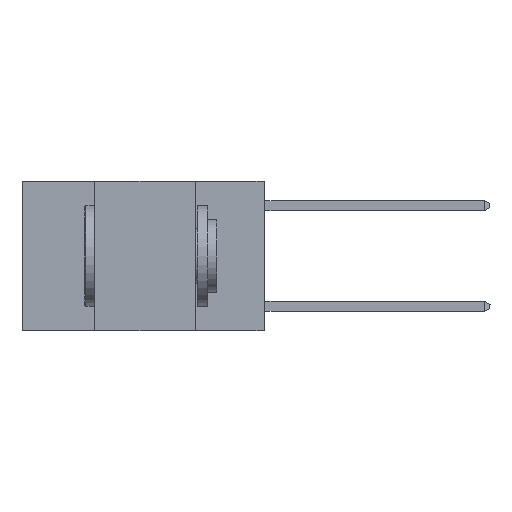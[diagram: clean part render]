
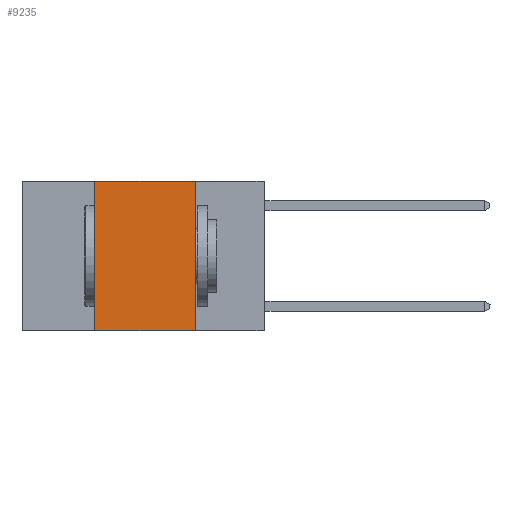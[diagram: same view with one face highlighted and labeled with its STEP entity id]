
A CAD part, left-side view. The second image highlights one B-rep face of the part: STEP entity #9235.
In plain terms, the highlighted planar face has unit normal (-1, 0, 0).
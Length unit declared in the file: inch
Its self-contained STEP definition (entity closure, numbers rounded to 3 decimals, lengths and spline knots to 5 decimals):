
#98 = EDGE_CURVE ( 'NONE', #6766, #1127, #9783, .T. ) ;
#351 = FACE_OUTER_BOUND ( 'NONE', #1460, .T. ) ;
#511 = AXIS2_PLACEMENT_3D ( 'NONE', #10784, #1380, #8042 ) ;
#761 = DIRECTION ( 'NONE',  ( 0., 0., -1. ) ) ;
#954 = DIRECTION ( 'NONE',  ( 0., -1., 0. ) ) ;
#1127 = VERTEX_POINT ( 'NONE', #7878 ) ;
#1380 = DIRECTION ( 'NONE',  ( 1., 0., 0. ) ) ;
#1415 = LINE ( 'NONE', #3638, #8433 ) ;
#1460 = EDGE_LOOP ( 'NONE', ( #1484, #9955, #1472, #11058 ) ) ;
#1472 = ORIENTED_EDGE ( 'NONE', *, *, #12001, .F. ) ;
#1484 = ORIENTED_EDGE ( 'NONE', *, *, #2543, .F. ) ;
#1720 = LINE ( 'NONE', #3779, #11430 ) ;
#2193 = VECTOR ( 'NONE', #2731, 39.37008 ) ;
#2543 = EDGE_CURVE ( 'NONE', #1127, #4722, #1415, .T. ) ;
#2731 = DIRECTION ( 'NONE',  ( 0., -1., 0. ) ) ;
#3173 = DIRECTION ( 'NONE',  ( 0., 0., 1. ) ) ;
#3638 = CARTESIAN_POINT ( 'NONE',  ( 0., 0.17, 0. ) ) ;
#3779 = CARTESIAN_POINT ( 'NONE',  ( 0., 0.6, -0.37 ) ) ;
#4722 = VERTEX_POINT ( 'NONE', #6470 ) ;
#4983 = VERTEX_POINT ( 'NONE', #5002 ) ;
#5002 = CARTESIAN_POINT ( 'NONE',  ( 0., 0.42, -0.37 ) ) ;
#6038 = CARTESIAN_POINT ( 'NONE',  ( 0., 0.42, 0. ) ) ;
#6237 = CARTESIAN_POINT ( 'NONE',  ( 0., 0.6, 0. ) ) ;
#6470 = CARTESIAN_POINT ( 'NONE',  ( 0., 0.17, -0.37 ) ) ;
#6766 = VERTEX_POINT ( 'NONE', #10088 ) ;
#7103 = PLANE ( 'NONE',  #511 ) ;
#7824 = VECTOR ( 'NONE', #3173, 39.37008 ) ;
#7878 = CARTESIAN_POINT ( 'NONE',  ( 0., 0.17, 0. ) ) ;
#8042 = DIRECTION ( 'NONE',  ( 0., 0., -1. ) ) ;
#8123 = LINE ( 'NONE', #6038, #7824 ) ;
#8433 = VECTOR ( 'NONE', #761, 39.37008 ) ;
#8481 = EDGE_CURVE ( 'NONE', #4983, #4722, #1720, .T. ) ;
#9235 = ADVANCED_FACE ( 'NONE', ( #351 ), #7103, .F. ) ;
#9783 = LINE ( 'NONE', #6237, #2193 ) ;
#9955 = ORIENTED_EDGE ( 'NONE', *, *, #98, .F. ) ;
#10088 = CARTESIAN_POINT ( 'NONE',  ( 0., 0.42, 0. ) ) ;
#10784 = CARTESIAN_POINT ( 'NONE',  ( 0., 0.6, 0. ) ) ;
#11058 = ORIENTED_EDGE ( 'NONE', *, *, #8481, .T. ) ;
#11430 = VECTOR ( 'NONE', #954, 39.37008 ) ;
#12001 = EDGE_CURVE ( 'NONE', #4983, #6766, #8123, .T. ) ;
